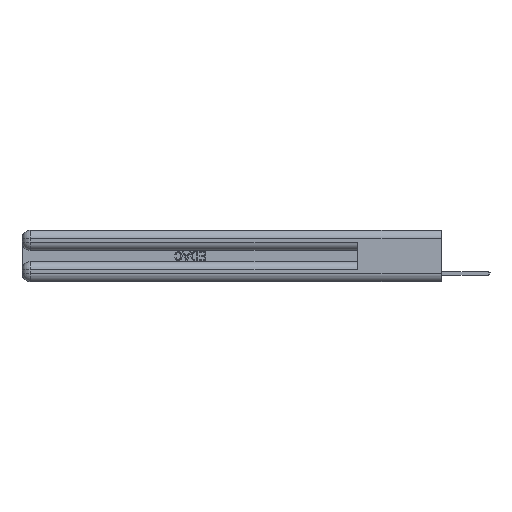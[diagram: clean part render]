
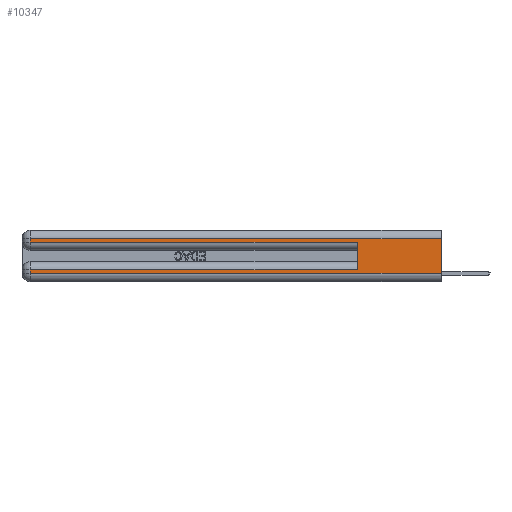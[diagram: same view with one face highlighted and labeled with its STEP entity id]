
A CAD part, left-side view. The second image highlights one B-rep face of the part: STEP entity #10347.
In plain terms, the highlighted planar face has unit normal (-1, 0, 0).
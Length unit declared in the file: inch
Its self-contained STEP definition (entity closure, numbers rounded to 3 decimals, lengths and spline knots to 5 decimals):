
#76 = VERTEX_POINT ( 'NONE', #1557 ) ;
#593 = EDGE_LOOP ( 'NONE', ( #9335, #30360, #6263, #7571, #9443, #28104, #29851, #11955 ) ) ;
#1557 = CARTESIAN_POINT ( 'NONE',  ( 0., 2.94, 0.31 ) ) ;
#1832 = VECTOR ( 'NONE', #9553, 39.37008 ) ;
#2892 = CARTESIAN_POINT ( 'NONE',  ( 0., 0., 0.37 ) ) ;
#3047 = EDGE_CURVE ( 'NONE', #29466, #6235, #29601, .T. ) ;
#3306 = VECTOR ( 'NONE', #17001, 39.37008 ) ;
#4202 = VECTOR ( 'NONE', #11228, 39.37008 ) ;
#4745 = DIRECTION ( 'NONE',  ( 0., -1., 0. ) ) ;
#4887 = EDGE_CURVE ( 'NONE', #25888, #32078, #26424, .T. ) ;
#5105 = CARTESIAN_POINT ( 'NONE',  ( 0., 0.6, 0.285 ) ) ;
#5506 = CARTESIAN_POINT ( 'NONE',  ( 0., 0., 0.31 ) ) ;
#5671 = LINE ( 'NONE', #20264, #32810 ) ;
#5754 = CARTESIAN_POINT ( 'NONE',  ( 0., 0.6, 0.145 ) ) ;
#6203 = CARTESIAN_POINT ( 'NONE',  ( 0., 2.94, 0.06 ) ) ;
#6235 = VERTEX_POINT ( 'NONE', #5105 ) ;
#6263 = ORIENTED_EDGE ( 'NONE', *, *, #7851, .T. ) ;
#7506 = EDGE_CURVE ( 'NONE', #32078, #16852, #13105, .T. ) ;
#7571 = ORIENTED_EDGE ( 'NONE', *, *, #3047, .T. ) ;
#7798 = EDGE_CURVE ( 'NONE', #30659, #17274, #28393, .T. ) ;
#7851 = EDGE_CURVE ( 'NONE', #76, #29466, #20351, .T. ) ;
#8190 = PLANE ( 'NONE',  #9801 ) ;
#8283 = CARTESIAN_POINT ( 'NONE',  ( 0., 2.94, 0.37 ) ) ;
#9335 = ORIENTED_EDGE ( 'NONE', *, *, #7798, .F. ) ;
#9443 = ORIENTED_EDGE ( 'NONE', *, *, #28696, .F. ) ;
#9518 = LINE ( 'NONE', #5754, #1832 ) ;
#9553 = DIRECTION ( 'NONE',  ( 0., 0., 1. ) ) ;
#9801 = AXIS2_PLACEMENT_3D ( 'NONE', #34820, #35023, #18259 ) ;
#10208 = EDGE_CURVE ( 'NONE', #30659, #76, #26461, .T. ) ;
#10347 = ADVANCED_FACE ( 'NONE', ( #15788 ), #8190, .F. ) ;
#10420 = CARTESIAN_POINT ( 'NONE',  ( 0., 2.94, 0.37 ) ) ;
#11094 = DIRECTION ( 'NONE',  ( 0., 1., 0. ) ) ;
#11121 = CARTESIAN_POINT ( 'NONE',  ( 0., 0., 0.06 ) ) ;
#11228 = DIRECTION ( 'NONE',  ( 0., 0., -1. ) ) ;
#11955 = ORIENTED_EDGE ( 'NONE', *, *, #13814, .T. ) ;
#12015 = VECTOR ( 'NONE', #13744, 39.37008 ) ;
#13105 = LINE ( 'NONE', #8283, #4202 ) ;
#13744 = DIRECTION ( 'NONE',  ( 0., 1., 0. ) ) ;
#13814 = EDGE_CURVE ( 'NONE', #16852, #17274, #5671, .T. ) ;
#13923 = VECTOR ( 'NONE', #21936, 39.37008 ) ;
#14168 = CARTESIAN_POINT ( 'NONE',  ( 0., 2.94, 0.085 ) ) ;
#14644 = CARTESIAN_POINT ( 'NONE',  ( 0., 2.94, 0.285 ) ) ;
#15788 = FACE_OUTER_BOUND ( 'NONE', #593, .T. ) ;
#16574 = CARTESIAN_POINT ( 'NONE',  ( 0., 0., 0.31 ) ) ;
#16852 = VERTEX_POINT ( 'NONE', #6203 ) ;
#17001 = DIRECTION ( 'NONE',  ( 0., -1., 0. ) ) ;
#17274 = VERTEX_POINT ( 'NONE', #11121 ) ;
#18259 = DIRECTION ( 'NONE',  ( 0., 0., -1. ) ) ;
#20264 = CARTESIAN_POINT ( 'NONE',  ( 0., 0., 0.06 ) ) ;
#20351 = LINE ( 'NONE', #10420, #32998 ) ;
#21110 = DIRECTION ( 'NONE',  ( 0., 0., -1. ) ) ;
#21936 = DIRECTION ( 'NONE',  ( 0., 0., -1. ) ) ;
#22493 = CARTESIAN_POINT ( 'NONE',  ( 0., 0., 0.285 ) ) ;
#25888 = VERTEX_POINT ( 'NONE', #26077 ) ;
#26077 = CARTESIAN_POINT ( 'NONE',  ( 0., 0.6, 0.085 ) ) ;
#26424 = LINE ( 'NONE', #34637, #12015 ) ;
#26461 = LINE ( 'NONE', #5506, #29019 ) ;
#28104 = ORIENTED_EDGE ( 'NONE', *, *, #4887, .T. ) ;
#28393 = LINE ( 'NONE', #2892, #13923 ) ;
#28696 = EDGE_CURVE ( 'NONE', #25888, #6235, #9518, .T. ) ;
#29019 = VECTOR ( 'NONE', #11094, 39.37008 ) ;
#29466 = VERTEX_POINT ( 'NONE', #14644 ) ;
#29601 = LINE ( 'NONE', #22493, #3306 ) ;
#29851 = ORIENTED_EDGE ( 'NONE', *, *, #7506, .T. ) ;
#30360 = ORIENTED_EDGE ( 'NONE', *, *, #10208, .T. ) ;
#30659 = VERTEX_POINT ( 'NONE', #16574 ) ;
#32078 = VERTEX_POINT ( 'NONE', #14168 ) ;
#32810 = VECTOR ( 'NONE', #4745, 39.37008 ) ;
#32998 = VECTOR ( 'NONE', #21110, 39.37008 ) ;
#34637 = CARTESIAN_POINT ( 'NONE',  ( 0., 0., 0.085 ) ) ;
#34820 = CARTESIAN_POINT ( 'NONE',  ( 0., 0., 0.37 ) ) ;
#35023 = DIRECTION ( 'NONE',  ( 1., 0., 0. ) ) ;
